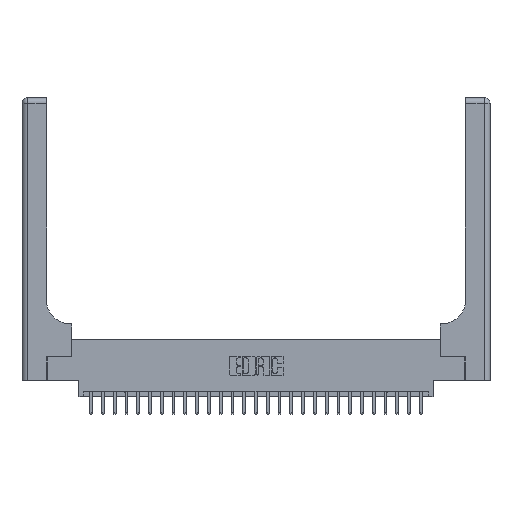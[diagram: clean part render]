
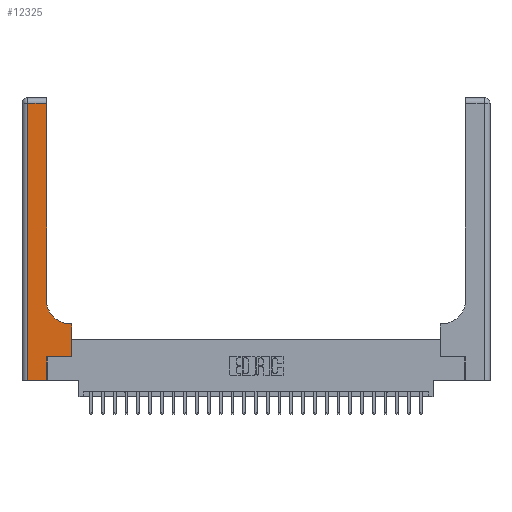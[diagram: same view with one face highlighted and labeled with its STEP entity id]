
A CAD part, top view. The second image highlights one B-rep face of the part: STEP entity #12325.
In plain terms, the highlighted planar face has unit normal (0, 0, 1).
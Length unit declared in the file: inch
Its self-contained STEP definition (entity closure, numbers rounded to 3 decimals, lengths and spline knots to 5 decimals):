
#1 = LINE ( 'NONE', #12296, #5818 ) ;
#7 = DIRECTION ( 'NONE',  ( 0., 0., -1. ) ) ;
#268 = FACE_OUTER_BOUND ( 'NONE', #7946, .T. ) ;
#758 = DIRECTION ( 'NONE',  ( 1., 0., 0. ) ) ;
#949 = VERTEX_POINT ( 'NONE', #14449 ) ;
#1767 = EDGE_CURVE ( 'NONE', #9617, #6854, #22397, .T. ) ;
#2193 = EDGE_CURVE ( 'NONE', #25704, #20226, #10470, .T. ) ;
#2655 = CARTESIAN_POINT ( 'NONE',  ( 0.265, 0., 0.37 ) ) ;
#2973 = LINE ( 'NONE', #7000, #7449 ) ;
#3266 = ORIENTED_EDGE ( 'NONE', *, *, #25093, .T. ) ;
#3954 = DIRECTION ( 'NONE',  ( -1., 0., 0. ) ) ;
#4262 = LINE ( 'NONE', #16777, #5195 ) ;
#4735 = VERTEX_POINT ( 'NONE', #20838 ) ;
#5195 = VECTOR ( 'NONE', #12474, 39.37008 ) ;
#5818 = VECTOR ( 'NONE', #10017, 39.37008 ) ;
#5964 = CARTESIAN_POINT ( 'NONE',  ( 0., 3., 0.37 ) ) ;
#6314 = ORIENTED_EDGE ( 'NONE', *, *, #2193, .T. ) ;
#6854 = VERTEX_POINT ( 'NONE', #13936 ) ;
#6939 = CARTESIAN_POINT ( 'NONE',  ( 0.528, 0.6, 0.37 ) ) ;
#7000 = CARTESIAN_POINT ( 'NONE',  ( 0.265, 0.25, 0.37 ) ) ;
#7302 = EDGE_CURVE ( 'NONE', #4735, #15992, #21077, .T. ) ;
#7449 = VECTOR ( 'NONE', #23415, 39.37008 ) ;
#7624 = ORIENTED_EDGE ( 'NONE', *, *, #7302, .T. ) ;
#7946 = EDGE_LOOP ( 'NONE', ( #17904, #3266, #7624, #21158, #6314, #18813, #10649, #19117, #16183 ) ) ;
#8069 = CARTESIAN_POINT ( 'NONE',  ( 0.51, 0.85, 0.37 ) ) ;
#8361 = VERTEX_POINT ( 'NONE', #14979 ) ;
#9617 = VERTEX_POINT ( 'NONE', #17414 ) ;
#9924 = EDGE_CURVE ( 'NONE', #15992, #25704, #19339, .T. ) ;
#10017 = DIRECTION ( 'NONE',  ( -1., 0., 0. ) ) ;
#10470 = LINE ( 'NONE', #16380, #16852 ) ;
#10649 = ORIENTED_EDGE ( 'NONE', *, *, #24349, .T. ) ;
#11449 = CARTESIAN_POINT ( 'NONE',  ( 0., 0., 0.37 ) ) ;
#12296 = CARTESIAN_POINT ( 'NONE',  ( 0., 2.94, 0.37 ) ) ;
#12325 = ADVANCED_FACE ( 'NONE', ( #268 ), #14433, .F. ) ;
#12474 = DIRECTION ( 'NONE',  ( 0., 1., 0. ) ) ;
#12506 = CARTESIAN_POINT ( 'NONE',  ( 0.06, 0., 0.37 ) ) ;
#12654 = DIRECTION ( 'NONE',  ( 0., 0., -1. ) ) ;
#13016 = AXIS2_PLACEMENT_3D ( 'NONE', #5964, #7, #3954 ) ;
#13275 = LINE ( 'NONE', #18933, #23357 ) ;
#13405 = AXIS2_PLACEMENT_3D ( 'NONE', #8069, #12654, #18157 ) ;
#13936 = CARTESIAN_POINT ( 'NONE',  ( 0.26, 0.85, 0.37 ) ) ;
#14122 = CARTESIAN_POINT ( 'NONE',  ( 0.26, 0.6, 0.37 ) ) ;
#14433 = PLANE ( 'NONE',  #13016 ) ;
#14449 = CARTESIAN_POINT ( 'NONE',  ( 0.528, 0.25, 0.37 ) ) ;
#14911 = CARTESIAN_POINT ( 'NONE',  ( 0.06, 3., 0.37 ) ) ;
#14979 = CARTESIAN_POINT ( 'NONE',  ( 0.26, 2.94, 0.37 ) ) ;
#15992 = VERTEX_POINT ( 'NONE', #12506 ) ;
#16183 = ORIENTED_EDGE ( 'NONE', *, *, #1767, .T. ) ;
#16380 = CARTESIAN_POINT ( 'NONE',  ( 0.265, 0., 0.37 ) ) ;
#16397 = EDGE_CURVE ( 'NONE', #6854, #8361, #4262, .T. ) ;
#16650 = DIRECTION ( 'NONE',  ( 0., 1., 0. ) ) ;
#16777 = CARTESIAN_POINT ( 'NONE',  ( 0.26, 3., 0.37 ) ) ;
#16852 = VECTOR ( 'NONE', #16650, 39.37008 ) ;
#16919 = DIRECTION ( 'NONE',  ( 0., 1., 0. ) ) ;
#17414 = CARTESIAN_POINT ( 'NONE',  ( 0.51, 0.6, 0.37 ) ) ;
#17832 = VERTEX_POINT ( 'NONE', #6939 ) ;
#17904 = ORIENTED_EDGE ( 'NONE', *, *, #16397, .T. ) ;
#18157 = DIRECTION ( 'NONE',  ( 1., 0., 0. ) ) ;
#18530 = VECTOR ( 'NONE', #20527, 39.37008 ) ;
#18813 = ORIENTED_EDGE ( 'NONE', *, *, #23403, .T. ) ;
#18933 = CARTESIAN_POINT ( 'NONE',  ( 0.528, 0.25, 0.37 ) ) ;
#19117 = ORIENTED_EDGE ( 'NONE', *, *, #19229, .T. ) ;
#19229 = EDGE_CURVE ( 'NONE', #17832, #9617, #26305, .T. ) ;
#19339 = LINE ( 'NONE', #11449, #24020 ) ;
#20226 = VERTEX_POINT ( 'NONE', #21501 ) ;
#20527 = DIRECTION ( 'NONE',  ( -1., 0., 0. ) ) ;
#20838 = CARTESIAN_POINT ( 'NONE',  ( 0.06, 2.94, 0.37 ) ) ;
#21077 = LINE ( 'NONE', #14911, #21352 ) ;
#21158 = ORIENTED_EDGE ( 'NONE', *, *, #9924, .T. ) ;
#21219 = DIRECTION ( 'NONE',  ( 0., -1., 0. ) ) ;
#21352 = VECTOR ( 'NONE', #21219, 39.37008 ) ;
#21501 = CARTESIAN_POINT ( 'NONE',  ( 0.265, 0.25, 0.37 ) ) ;
#22397 = CIRCLE ( 'NONE', #13405, 0.25 ) ;
#23357 = VECTOR ( 'NONE', #16919, 39.37008 ) ;
#23403 = EDGE_CURVE ( 'NONE', #20226, #949, #2973, .T. ) ;
#23415 = DIRECTION ( 'NONE',  ( 1., 0., 0. ) ) ;
#24020 = VECTOR ( 'NONE', #758, 39.37008 ) ;
#24349 = EDGE_CURVE ( 'NONE', #949, #17832, #13275, .T. ) ;
#25093 = EDGE_CURVE ( 'NONE', #8361, #4735, #1, .T. ) ;
#25704 = VERTEX_POINT ( 'NONE', #2655 ) ;
#26305 = LINE ( 'NONE', #14122, #18530 ) ;
